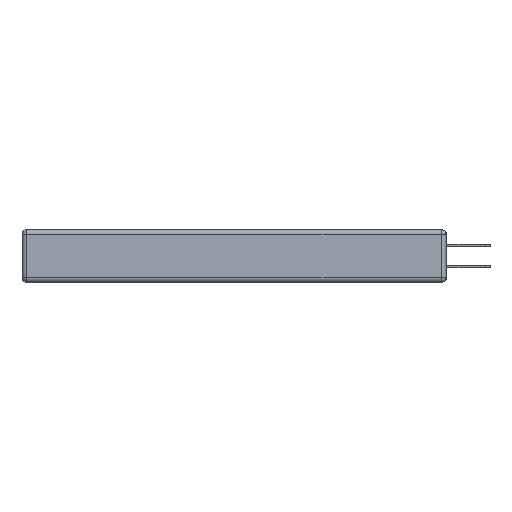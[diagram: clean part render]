
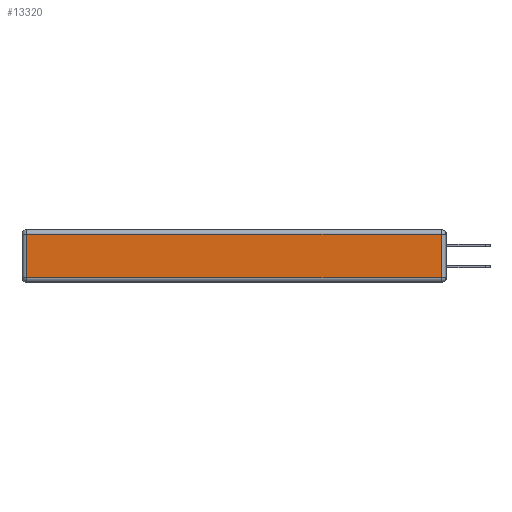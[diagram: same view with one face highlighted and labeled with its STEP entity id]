
A CAD part, left-side view. The second image highlights one B-rep face of the part: STEP entity #13320.
In plain terms, the highlighted planar face has unit normal (-1, 0, 0).
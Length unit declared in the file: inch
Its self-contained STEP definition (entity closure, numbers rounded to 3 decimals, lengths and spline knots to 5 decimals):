
#201 = AXIS2_PLACEMENT_3D ( 'NONE', #14437, #447, #11974 ) ;
#259 = DIRECTION ( 'NONE',  ( 0., 1., 0. ) ) ;
#279 = CARTESIAN_POINT ( 'NONE',  ( 0., 2.72, -0.313 ) ) ;
#447 = DIRECTION ( 'NONE',  ( -1., 0., 0. ) ) ;
#849 = VERTEX_POINT ( 'NONE', #15452 ) ;
#1617 = ORIENTED_EDGE ( 'NONE', *, *, #9148, .T. ) ;
#2062 = CARTESIAN_POINT ( 'NONE',  ( 0., 0.03, -0.343 ) ) ;
#2988 = CARTESIAN_POINT ( 'NONE',  ( 0., 2.75, -0.03 ) ) ;
#4181 = CARTESIAN_POINT ( 'NONE',  ( 0., 2.72, -0.343 ) ) ;
#5127 = VECTOR ( 'NONE', #259, 39.37008 ) ;
#5172 = ORIENTED_EDGE ( 'NONE', *, *, #14666, .T. ) ;
#6909 = VECTOR ( 'NONE', #10251, 39.37008 ) ;
#7238 = EDGE_LOOP ( 'NONE', ( #1617, #5172, #12573, #13859 ) ) ;
#8114 = PLANE ( 'NONE',  #201 ) ;
#8272 = EDGE_CURVE ( 'NONE', #16070, #9363, #8808, .T. ) ;
#8756 = LINE ( 'NONE', #8970, #16547 ) ;
#8808 = LINE ( 'NONE', #2988, #5127 ) ;
#8970 = CARTESIAN_POINT ( 'NONE',  ( 0., 0., -0.313 ) ) ;
#9148 = EDGE_CURVE ( 'NONE', #16305, #849, #8756, .T. ) ;
#9183 = FACE_OUTER_BOUND ( 'NONE', #7238, .T. ) ;
#9363 = VERTEX_POINT ( 'NONE', #10453 ) ;
#10041 = CARTESIAN_POINT ( 'NONE',  ( 0., 0.03, -0.03 ) ) ;
#10251 = DIRECTION ( 'NONE',  ( 0., 0., 1. ) ) ;
#10453 = CARTESIAN_POINT ( 'NONE',  ( 0., 2.72, -0.03 ) ) ;
#10529 = LINE ( 'NONE', #2062, #6909 ) ;
#11960 = VECTOR ( 'NONE', #13104, 39.37008 ) ;
#11974 = DIRECTION ( 'NONE',  ( 0., 0., 1. ) ) ;
#12573 = ORIENTED_EDGE ( 'NONE', *, *, #8272, .T. ) ;
#13104 = DIRECTION ( 'NONE',  ( 0., 0., -1. ) ) ;
#13163 = LINE ( 'NONE', #4181, #11960 ) ;
#13320 = ADVANCED_FACE ( 'NONE', ( #9183 ), #8114, .T. ) ;
#13859 = ORIENTED_EDGE ( 'NONE', *, *, #13951, .T. ) ;
#13951 = EDGE_CURVE ( 'NONE', #9363, #16305, #13163, .T. ) ;
#14437 = CARTESIAN_POINT ( 'NONE',  ( 0., 0., -0.343 ) ) ;
#14666 = EDGE_CURVE ( 'NONE', #849, #16070, #10529, .T. ) ;
#14747 = DIRECTION ( 'NONE',  ( 0., -1., 0. ) ) ;
#15452 = CARTESIAN_POINT ( 'NONE',  ( 0., 0.03, -0.313 ) ) ;
#16070 = VERTEX_POINT ( 'NONE', #10041 ) ;
#16305 = VERTEX_POINT ( 'NONE', #279 ) ;
#16547 = VECTOR ( 'NONE', #14747, 39.37008 ) ;
